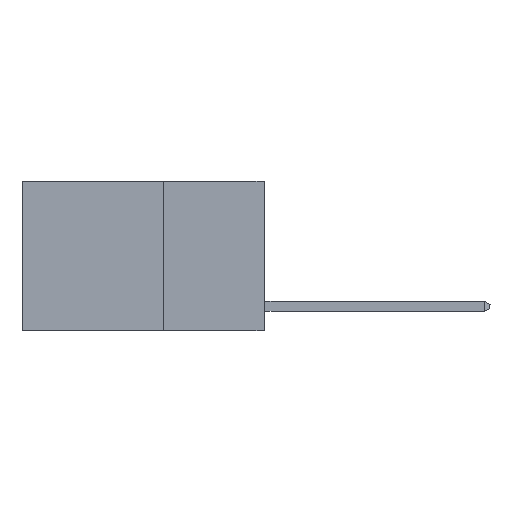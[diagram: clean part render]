
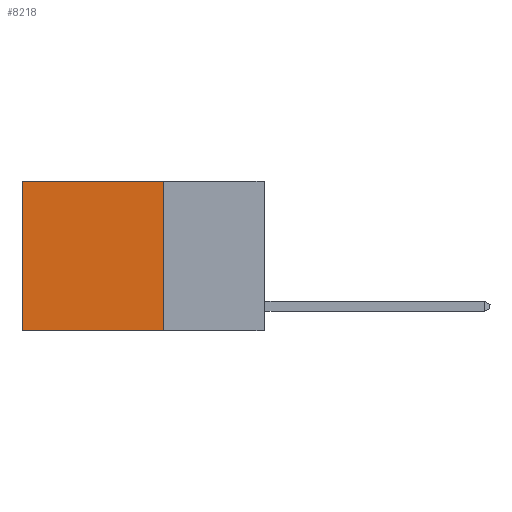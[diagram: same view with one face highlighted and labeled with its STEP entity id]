
A CAD part, left-side view. The second image highlights one B-rep face of the part: STEP entity #8218.
In plain terms, the highlighted planar face has unit normal (-1, 0, 0).
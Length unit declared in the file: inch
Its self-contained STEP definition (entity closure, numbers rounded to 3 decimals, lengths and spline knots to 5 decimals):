
#1044 = DIRECTION ( 'NONE',  ( 0., 0., -1. ) ) ;
#1733 = EDGE_CURVE ( 'NONE', #3904, #17779, #11320, .T. ) ;
#2353 = ORIENTED_EDGE ( 'NONE', *, *, #1733, .T. ) ;
#2393 = VERTEX_POINT ( 'NONE', #16043 ) ;
#3072 = EDGE_LOOP ( 'NONE', ( #8697, #24951, #16651, #2353 ) ) ;
#3904 = VERTEX_POINT ( 'NONE', #8919 ) ;
#4063 = CARTESIAN_POINT ( 'NONE',  ( 0.2625, 0.6, 0. ) ) ;
#6804 = CARTESIAN_POINT ( 'NONE',  ( 0.2625, 0.25, 0. ) ) ;
#7470 = PLANE ( 'NONE',  #21799 ) ;
#7742 = EDGE_CURVE ( 'NONE', #2393, #23970, #14028, .T. ) ;
#8006 = EDGE_CURVE ( 'NONE', #3904, #2393, #13089, .T. ) ;
#8218 = ADVANCED_FACE ( 'NONE', ( #11548 ), #7470, .F. ) ;
#8697 = ORIENTED_EDGE ( 'NONE', *, *, #12322, .T. ) ;
#8865 = DIRECTION ( 'NONE',  ( 0., 0., -1. ) ) ;
#8919 = CARTESIAN_POINT ( 'NONE',  ( 0.2625, 0.25, 0. ) ) ;
#10104 = VECTOR ( 'NONE', #21716, 39.37008 ) ;
#11247 = VECTOR ( 'NONE', #1044, 39.37008 ) ;
#11320 = LINE ( 'NONE', #17847, #10104 ) ;
#11350 = CARTESIAN_POINT ( 'NONE',  ( 0.2625, 0.25, 0. ) ) ;
#11548 = FACE_OUTER_BOUND ( 'NONE', #3072, .T. ) ;
#11725 = DIRECTION ( 'NONE',  ( 0., 1., 0. ) ) ;
#12322 = EDGE_CURVE ( 'NONE', #17779, #23970, #15386, .T. ) ;
#13089 = LINE ( 'NONE', #6804, #11247 ) ;
#13312 = DIRECTION ( 'NONE',  ( 0., 0., -1. ) ) ;
#14028 = LINE ( 'NONE', #15654, #23083 ) ;
#15386 = LINE ( 'NONE', #20471, #21132 ) ;
#15654 = CARTESIAN_POINT ( 'NONE',  ( 0.2625, 0.25, -0.37 ) ) ;
#16043 = CARTESIAN_POINT ( 'NONE',  ( 0.2625, 0.25, -0.37 ) ) ;
#16651 = ORIENTED_EDGE ( 'NONE', *, *, #8006, .F. ) ;
#17779 = VERTEX_POINT ( 'NONE', #4063 ) ;
#17847 = CARTESIAN_POINT ( 'NONE',  ( 0.2625, 0.25, 0. ) ) ;
#20471 = CARTESIAN_POINT ( 'NONE',  ( 0.2625, 0.6, 0. ) ) ;
#21084 = CARTESIAN_POINT ( 'NONE',  ( 0.2625, 0.6, -0.37 ) ) ;
#21132 = VECTOR ( 'NONE', #8865, 39.37008 ) ;
#21716 = DIRECTION ( 'NONE',  ( 0., 1., 0. ) ) ;
#21799 = AXIS2_PLACEMENT_3D ( 'NONE', #11350, #24881, #13312 ) ;
#23083 = VECTOR ( 'NONE', #11725, 39.37008 ) ;
#23970 = VERTEX_POINT ( 'NONE', #21084 ) ;
#24881 = DIRECTION ( 'NONE',  ( 1., 0., 0. ) ) ;
#24951 = ORIENTED_EDGE ( 'NONE', *, *, #7742, .F. ) ;
